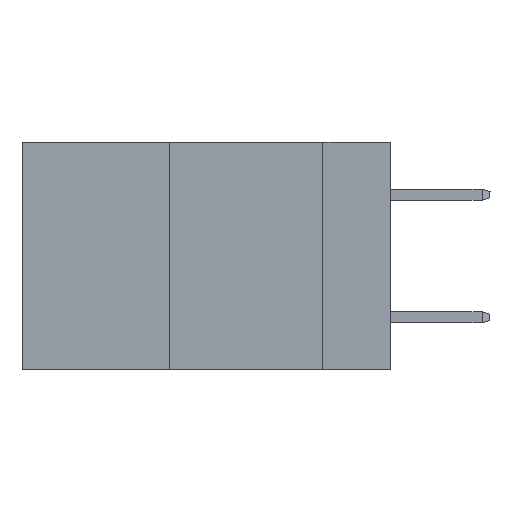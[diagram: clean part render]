
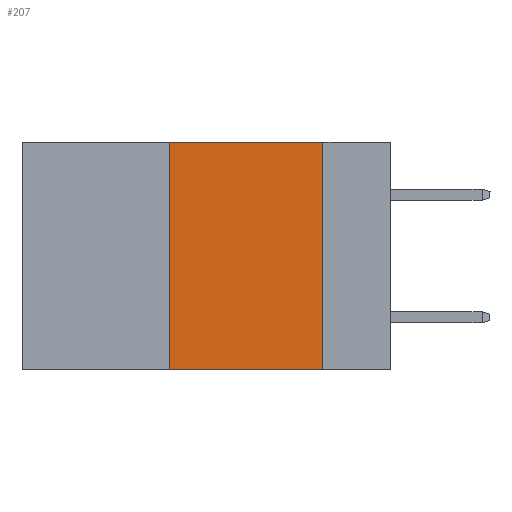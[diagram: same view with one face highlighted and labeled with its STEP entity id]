
A CAD part, left-side view. The second image highlights one B-rep face of the part: STEP entity #207.
In plain terms, the highlighted planar face has unit normal (-1, 0, 0).
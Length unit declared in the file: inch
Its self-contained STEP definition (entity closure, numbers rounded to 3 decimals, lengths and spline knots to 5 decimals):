
#94 = DIRECTION ( 'NONE',  ( 0., 0., 1. ) ) ;
#207 = ADVANCED_FACE ( 'NONE', ( #20634 ), #21320, .F. ) ;
#608 = ORIENTED_EDGE ( 'NONE', *, *, #10979, .F. ) ;
#1251 = LINE ( 'NONE', #13041, #11963 ) ;
#3661 = DIRECTION ( 'NONE',  ( 0., -1., 0. ) ) ;
#3910 = DIRECTION ( 'NONE',  ( 1., 0., 0. ) ) ;
#4619 = DIRECTION ( 'NONE',  ( 0., 0., -1. ) ) ;
#5383 = CARTESIAN_POINT ( 'NONE',  ( 0., 0.11, 0. ) ) ;
#5950 = EDGE_LOOP ( 'NONE', ( #22205, #9986, #608, #21751 ) ) ;
#5970 = DIRECTION ( 'NONE',  ( 0., 0., -1. ) ) ;
#6456 = VECTOR ( 'NONE', #3661, 39.37008 ) ;
#7522 = VERTEX_POINT ( 'NONE', #21558 ) ;
#7622 = CARTESIAN_POINT ( 'NONE',  ( 0., 0.11, -0.37 ) ) ;
#7771 = LINE ( 'NONE', #5383, #13325 ) ;
#8808 = CARTESIAN_POINT ( 'NONE',  ( 0., 0.6, -0.37 ) ) ;
#8947 = VERTEX_POINT ( 'NONE', #18862 ) ;
#8997 = EDGE_CURVE ( 'NONE', #24471, #13601, #17490, .T. ) ;
#9986 = ORIENTED_EDGE ( 'NONE', *, *, #14968, .F. ) ;
#10476 = AXIS2_PLACEMENT_3D ( 'NONE', #19622, #3910, #5970 ) ;
#10632 = VECTOR ( 'NONE', #94, 39.37008 ) ;
#10979 = EDGE_CURVE ( 'NONE', #24471, #7522, #19853, .T. ) ;
#11002 = DIRECTION ( 'NONE',  ( 0., -1., 0. ) ) ;
#11956 = CARTESIAN_POINT ( 'NONE',  ( 0., 0.36, -0.37 ) ) ;
#11963 = VECTOR ( 'NONE', #11002, 39.37008 ) ;
#13041 = CARTESIAN_POINT ( 'NONE',  ( 0., 0.6, 0. ) ) ;
#13143 = EDGE_CURVE ( 'NONE', #8947, #13601, #7771, .T. ) ;
#13325 = VECTOR ( 'NONE', #4619, 39.37008 ) ;
#13601 = VERTEX_POINT ( 'NONE', #7622 ) ;
#14968 = EDGE_CURVE ( 'NONE', #7522, #8947, #1251, .T. ) ;
#17490 = LINE ( 'NONE', #8808, #6456 ) ;
#18862 = CARTESIAN_POINT ( 'NONE',  ( 0., 0.11, 0. ) ) ;
#19622 = CARTESIAN_POINT ( 'NONE',  ( 0., 0.6, 0. ) ) ;
#19853 = LINE ( 'NONE', #21706, #10632 ) ;
#20634 = FACE_OUTER_BOUND ( 'NONE', #5950, .T. ) ;
#21320 = PLANE ( 'NONE',  #10476 ) ;
#21558 = CARTESIAN_POINT ( 'NONE',  ( 0., 0.36, 0. ) ) ;
#21706 = CARTESIAN_POINT ( 'NONE',  ( 0., 0.36, 0. ) ) ;
#21751 = ORIENTED_EDGE ( 'NONE', *, *, #8997, .T. ) ;
#22205 = ORIENTED_EDGE ( 'NONE', *, *, #13143, .F. ) ;
#24471 = VERTEX_POINT ( 'NONE', #11956 ) ;
